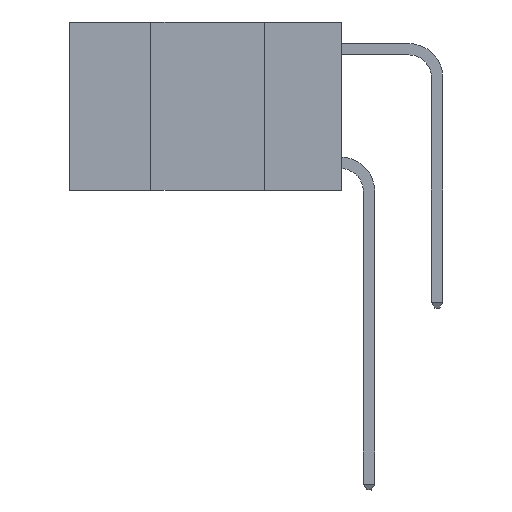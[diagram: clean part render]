
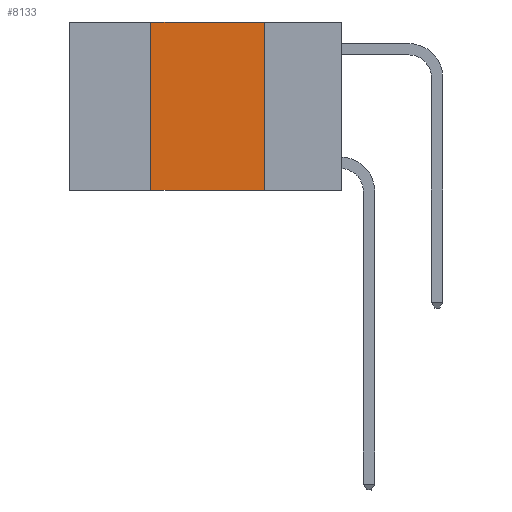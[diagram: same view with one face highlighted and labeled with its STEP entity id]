
A CAD part, left-side view. The second image highlights one B-rep face of the part: STEP entity #8133.
In plain terms, the highlighted planar face has unit normal (-1, 0, 0).
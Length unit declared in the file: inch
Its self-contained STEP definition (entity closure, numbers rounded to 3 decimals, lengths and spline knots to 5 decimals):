
#1663 = PLANE ( 'NONE',  #2999 ) ;
#1744 = CARTESIAN_POINT ( 'NONE',  ( 0., 0.6, 0. ) ) ;
#2228 = EDGE_CURVE ( 'NONE', #7520, #9035, #12861, .T. ) ;
#2420 = ORIENTED_EDGE ( 'NONE', *, *, #22732, .F. ) ;
#2999 = AXIS2_PLACEMENT_3D ( 'NONE', #1744, #14662, #3558 ) ;
#3546 = ORIENTED_EDGE ( 'NONE', *, *, #3888, .F. ) ;
#3549 = EDGE_LOOP ( 'NONE', ( #2420, #12309, #3546, #23002 ) ) ;
#3558 = DIRECTION ( 'NONE',  ( 0., 0., -1. ) ) ;
#3674 = LINE ( 'NONE', #6204, #22553 ) ;
#3888 = EDGE_CURVE ( 'NONE', #7038, #7520, #20359, .T. ) ;
#6020 = VERTEX_POINT ( 'NONE', #16149 ) ;
#6204 = CARTESIAN_POINT ( 'NONE',  ( 0., 0.6, -0.37 ) ) ;
#7038 = VERTEX_POINT ( 'NONE', #15414 ) ;
#7520 = VERTEX_POINT ( 'NONE', #16564 ) ;
#7949 = VECTOR ( 'NONE', #18062, 39.37008 ) ;
#8133 = ADVANCED_FACE ( 'NONE', ( #19389 ), #1663, .F. ) ;
#8739 = VECTOR ( 'NONE', #22402, 39.37008 ) ;
#9035 = VERTEX_POINT ( 'NONE', #11454 ) ;
#11454 = CARTESIAN_POINT ( 'NONE',  ( 0., 0.17, 0. ) ) ;
#12309 = ORIENTED_EDGE ( 'NONE', *, *, #2228, .F. ) ;
#12616 = CARTESIAN_POINT ( 'NONE',  ( 0., 0.6, 0. ) ) ;
#12861 = LINE ( 'NONE', #12616, #7949 ) ;
#13678 = DIRECTION ( 'NONE',  ( 0., -1., 0. ) ) ;
#14662 = DIRECTION ( 'NONE',  ( 1., 0., 0. ) ) ;
#15414 = CARTESIAN_POINT ( 'NONE',  ( 0., 0.42, -0.37 ) ) ;
#15588 = DIRECTION ( 'NONE',  ( 0., 0., 1. ) ) ;
#15613 = VECTOR ( 'NONE', #15588, 39.37008 ) ;
#16149 = CARTESIAN_POINT ( 'NONE',  ( 0., 0.17, -0.37 ) ) ;
#16564 = CARTESIAN_POINT ( 'NONE',  ( 0., 0.42, 0. ) ) ;
#17154 = CARTESIAN_POINT ( 'NONE',  ( 0., 0.42, 0. ) ) ;
#18062 = DIRECTION ( 'NONE',  ( 0., -1., 0. ) ) ;
#18662 = EDGE_CURVE ( 'NONE', #7038, #6020, #3674, .T. ) ;
#19389 = FACE_OUTER_BOUND ( 'NONE', #3549, .T. ) ;
#20359 = LINE ( 'NONE', #17154, #15613 ) ;
#20595 = CARTESIAN_POINT ( 'NONE',  ( 0., 0.17, 0. ) ) ;
#22402 = DIRECTION ( 'NONE',  ( 0., 0., -1. ) ) ;
#22553 = VECTOR ( 'NONE', #13678, 39.37008 ) ;
#22732 = EDGE_CURVE ( 'NONE', #9035, #6020, #23167, .T. ) ;
#23002 = ORIENTED_EDGE ( 'NONE', *, *, #18662, .T. ) ;
#23167 = LINE ( 'NONE', #20595, #8739 ) ;
